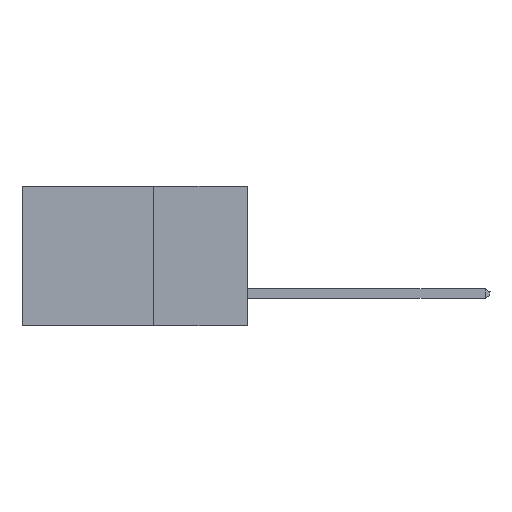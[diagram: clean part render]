
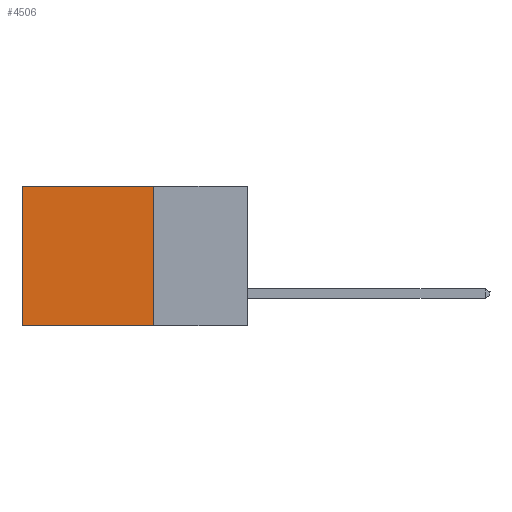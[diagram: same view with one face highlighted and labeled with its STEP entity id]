
A CAD part, left-side view. The second image highlights one B-rep face of the part: STEP entity #4506.
In plain terms, the highlighted planar face has unit normal (-1, 0, 0).
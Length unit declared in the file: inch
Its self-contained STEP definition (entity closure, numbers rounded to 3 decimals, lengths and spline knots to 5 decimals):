
#681 = CARTESIAN_POINT ( 'NONE',  ( 0.2615, 0.6, 0. ) ) ;
#1181 = LINE ( 'NONE', #2879, #2400 ) ;
#1274 = DIRECTION ( 'NONE',  ( 0., 0., -1. ) ) ;
#1846 = ORIENTED_EDGE ( 'NONE', *, *, #8855, .T. ) ;
#2400 = VECTOR ( 'NONE', #2681, 39.37008 ) ;
#2681 = DIRECTION ( 'NONE',  ( 0., 1., 0. ) ) ;
#2785 = EDGE_CURVE ( 'NONE', #6986, #7097, #7236, .T. ) ;
#2879 = CARTESIAN_POINT ( 'NONE',  ( 0.2615, 0.25, -0.37 ) ) ;
#2978 = CARTESIAN_POINT ( 'NONE',  ( 0.2615, 0.25, 0. ) ) ;
#4410 = LINE ( 'NONE', #2978, #11799 ) ;
#4506 = ADVANCED_FACE ( 'NONE', ( #16384 ), #5900, .F. ) ;
#5023 = VERTEX_POINT ( 'NONE', #7189 ) ;
#5255 = ORIENTED_EDGE ( 'NONE', *, *, #2785, .F. ) ;
#5900 = PLANE ( 'NONE',  #13597 ) ;
#5947 = VECTOR ( 'NONE', #11681, 39.37008 ) ;
#6433 = CARTESIAN_POINT ( 'NONE',  ( 0.2615, 0.25, -0.37 ) ) ;
#6986 = VERTEX_POINT ( 'NONE', #8887 ) ;
#7097 = VERTEX_POINT ( 'NONE', #6433 ) ;
#7189 = CARTESIAN_POINT ( 'NONE',  ( 0.2615, 0.6, -0.37 ) ) ;
#7236 = LINE ( 'NONE', #8963, #16441 ) ;
#7378 = EDGE_LOOP ( 'NONE', ( #1846, #10309, #5255, #13343 ) ) ;
#8549 = EDGE_CURVE ( 'NONE', #7097, #5023, #1181, .T. ) ;
#8750 = CARTESIAN_POINT ( 'NONE',  ( 0.2615, 0.25, -0.37 ) ) ;
#8855 = EDGE_CURVE ( 'NONE', #15244, #5023, #10072, .T. ) ;
#8887 = CARTESIAN_POINT ( 'NONE',  ( 0.2615, 0.25, 0. ) ) ;
#8963 = CARTESIAN_POINT ( 'NONE',  ( 0.2615, 0.25, -0.37 ) ) ;
#10072 = LINE ( 'NONE', #16190, #5947 ) ;
#10309 = ORIENTED_EDGE ( 'NONE', *, *, #8549, .F. ) ;
#10330 = EDGE_CURVE ( 'NONE', #6986, #15244, #4410, .T. ) ;
#11681 = DIRECTION ( 'NONE',  ( 0., 0., -1. ) ) ;
#11799 = VECTOR ( 'NONE', #17373, 39.37008 ) ;
#11967 = DIRECTION ( 'NONE',  ( 1., 0., 0. ) ) ;
#12068 = DIRECTION ( 'NONE',  ( 0., 0., -1. ) ) ;
#13343 = ORIENTED_EDGE ( 'NONE', *, *, #10330, .T. ) ;
#13597 = AXIS2_PLACEMENT_3D ( 'NONE', #8750, #11967, #12068 ) ;
#15244 = VERTEX_POINT ( 'NONE', #681 ) ;
#16190 = CARTESIAN_POINT ( 'NONE',  ( 0.2615, 0.6, -0.37 ) ) ;
#16384 = FACE_OUTER_BOUND ( 'NONE', #7378, .T. ) ;
#16441 = VECTOR ( 'NONE', #1274, 39.37008 ) ;
#17373 = DIRECTION ( 'NONE',  ( 0., 1., 0. ) ) ;
